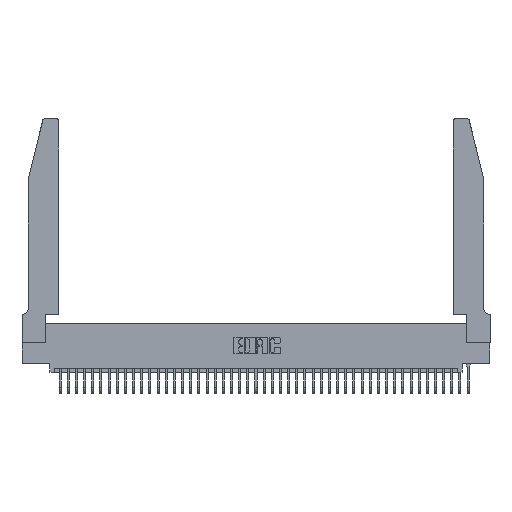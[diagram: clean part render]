
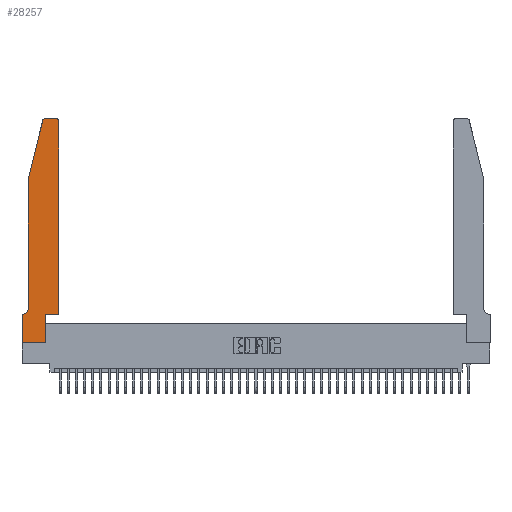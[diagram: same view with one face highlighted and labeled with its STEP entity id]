
A CAD part, top view. The second image highlights one B-rep face of the part: STEP entity #28257.
In plain terms, the highlighted planar face has unit normal (0, 0, 1).
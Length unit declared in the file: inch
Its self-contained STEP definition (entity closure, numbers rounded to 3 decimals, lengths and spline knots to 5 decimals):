
#70 = ORIENTED_EDGE ( 'NONE', *, *, #24352, .T. ) ;
#565 = ORIENTED_EDGE ( 'NONE', *, *, #25854, .T. ) ;
#1243 = VERTEX_POINT ( 'NONE', #2522 ) ;
#1568 = DIRECTION ( 'NONE',  ( 0., 0., 1. ) ) ;
#1955 = CARTESIAN_POINT ( 'NONE',  ( 0., 0., 0.37 ) ) ;
#2493 = VECTOR ( 'NONE', #31071, 39.37008 ) ;
#2522 = CARTESIAN_POINT ( 'NONE',  ( 0.4505, 2.72, 0.37 ) ) ;
#2600 = DIRECTION ( 'NONE',  ( 1., 0., 0. ) ) ;
#3411 = DIRECTION ( 'NONE',  ( 0., 0., -1. ) ) ;
#3461 = CARTESIAN_POINT ( 'NONE',  ( 0.0755, 0.42, 0.37 ) ) ;
#3515 = LINE ( 'NONE', #27961, #2493 ) ;
#3892 = VECTOR ( 'NONE', #11024, 39.37008 ) ;
#4000 = PLANE ( 'NONE',  #39865 ) ;
#5388 = VECTOR ( 'NONE', #6300, 39.37008 ) ;
#5618 = DIRECTION ( 'NONE',  ( 0., -1., 0. ) ) ;
#5879 = EDGE_CURVE ( 'NONE', #16688, #23984, #29863, .T. ) ;
#5885 = VECTOR ( 'NONE', #14058, 39.37008 ) ;
#6300 = DIRECTION ( 'NONE',  ( 1., 0., 0. ) ) ;
#7277 = DIRECTION ( 'NONE',  ( 0., 0., 1. ) ) ;
#7599 = CARTESIAN_POINT ( 'NONE',  ( 0.0755, 0.35, 0.37 ) ) ;
#7938 = EDGE_CURVE ( 'NONE', #16763, #21421, #29204, .T. ) ;
#8326 = ORIENTED_EDGE ( 'NONE', *, *, #30070, .T. ) ;
#8475 = LINE ( 'NONE', #40564, #25289 ) ;
#8668 = DIRECTION ( 'NONE',  ( 0., 1., 0. ) ) ;
#8767 = CARTESIAN_POINT ( 'NONE',  ( 0.0755, 2., 0.37 ) ) ;
#8951 = ORIENTED_EDGE ( 'NONE', *, *, #5879, .T. ) ;
#9298 = ORIENTED_EDGE ( 'NONE', *, *, #7938, .T. ) ;
#9329 = VERTEX_POINT ( 'NONE', #1955 ) ;
#10605 = VECTOR ( 'NONE', #2600, 39.37008 ) ;
#11024 = DIRECTION ( 'NONE',  ( -1., 0., 0. ) ) ;
#12360 = VECTOR ( 'NONE', #36499, 39.37008 ) ;
#12567 = EDGE_CURVE ( 'NONE', #26544, #14189, #13908, .T. ) ;
#13908 = LINE ( 'NONE', #8767, #30537 ) ;
#14058 = DIRECTION ( 'NONE',  ( 0., -1., 0. ) ) ;
#14189 = VERTEX_POINT ( 'NONE', #3461 ) ;
#14202 = VECTOR ( 'NONE', #8668, 39.37008 ) ;
#15134 = DIRECTION ( 'NONE',  ( 0., 0., 1. ) ) ;
#16160 = EDGE_CURVE ( 'NONE', #29964, #26544, #3515, .T. ) ;
#16688 = VERTEX_POINT ( 'NONE', #39646 ) ;
#16763 = VERTEX_POINT ( 'NONE', #27642 ) ;
#16911 = AXIS2_PLACEMENT_3D ( 'NONE', #20706, #1568, #23895 ) ;
#17182 = VERTEX_POINT ( 'NONE', #17239 ) ;
#17239 = CARTESIAN_POINT ( 'NONE',  ( 0.284, 2.75, 0.37 ) ) ;
#17277 = VERTEX_POINT ( 'NONE', #18311 ) ;
#18182 = CARTESIAN_POINT ( 'NONE',  ( 0.25487, 2.72718, 0.37 ) ) ;
#18311 = CARTESIAN_POINT ( 'NONE',  ( 0.4505, 0.35, 0.37 ) ) ;
#18695 = ORIENTED_EDGE ( 'NONE', *, *, #22180, .T. ) ;
#18732 = CARTESIAN_POINT ( 'NONE',  ( 0.4205, 2.75, 0.37 ) ) ;
#18925 = ORIENTED_EDGE ( 'NONE', *, *, #16160, .T. ) ;
#20449 = CARTESIAN_POINT ( 'NONE',  ( 0.0755, 2., 0.37 ) ) ;
#20580 = ORIENTED_EDGE ( 'NONE', *, *, #12567, .T. ) ;
#20706 = CARTESIAN_POINT ( 'NONE',  ( 0.284, 2.72, 0.37 ) ) ;
#20847 = CIRCLE ( 'NONE', #21564, 0.03 ) ;
#21421 = VERTEX_POINT ( 'NONE', #31385 ) ;
#21564 = AXIS2_PLACEMENT_3D ( 'NONE', #33845, #15134, #36988 ) ;
#21856 = DIRECTION ( 'NONE',  ( -1., 0., 0. ) ) ;
#22131 = CARTESIAN_POINT ( 'NONE',  ( 0.4505, 0.35, 0.37 ) ) ;
#22180 = EDGE_CURVE ( 'NONE', #1243, #30088, #20847, .T. ) ;
#22493 = CARTESIAN_POINT ( 'NONE',  ( 0.0055, 0.42, 0.37 ) ) ;
#22948 = CIRCLE ( 'NONE', #35762, 0.07 ) ;
#23326 = LINE ( 'NONE', #22131, #5388 ) ;
#23511 = CARTESIAN_POINT ( 'NONE',  ( 0., 0., 0.37 ) ) ;
#23895 = DIRECTION ( 'NONE',  ( 1., 0., 0. ) ) ;
#23984 = VERTEX_POINT ( 'NONE', #30187 ) ;
#24352 = EDGE_CURVE ( 'NONE', #14189, #16763, #22948, .T. ) ;
#24912 = CARTESIAN_POINT ( 'NONE',  ( 0., 0., 0.37 ) ) ;
#25289 = VECTOR ( 'NONE', #21856, 39.37008 ) ;
#25668 = DIRECTION ( 'NONE',  ( -1., 0., 0. ) ) ;
#25749 = EDGE_CURVE ( 'NONE', #30088, #17182, #8475, .T. ) ;
#25854 = EDGE_CURVE ( 'NONE', #23984, #17277, #23326, .T. ) ;
#25924 = EDGE_LOOP ( 'NONE', ( #37283, #27921, #18925, #20580, #70, #9298, #37052, #8326, #8951, #565, #35861, #18695 ) ) ;
#26044 = EDGE_CURVE ( 'NONE', #21421, #9329, #38443, .T. ) ;
#26286 = CIRCLE ( 'NONE', #16911, 0.03 ) ;
#26544 = VERTEX_POINT ( 'NONE', #20449 ) ;
#27544 = CARTESIAN_POINT ( 'NONE',  ( 0.2865, 0.35, 0.37 ) ) ;
#27642 = CARTESIAN_POINT ( 'NONE',  ( 0.0055, 0.35, 0.37 ) ) ;
#27810 = EDGE_CURVE ( 'NONE', #17277, #1243, #30019, .T. ) ;
#27921 = ORIENTED_EDGE ( 'NONE', *, *, #30973, .T. ) ;
#27961 = CARTESIAN_POINT ( 'NONE',  ( 0.0755, 2., 0.37 ) ) ;
#28257 = ADVANCED_FACE ( 'NONE', ( #36318 ), #4000, .T. ) ;
#28312 = LINE ( 'NONE', #24912, #10605 ) ;
#29204 = LINE ( 'NONE', #7599, #3892 ) ;
#29379 = DIRECTION ( 'NONE',  ( 1., 0., 0. ) ) ;
#29863 = LINE ( 'NONE', #27544, #14202 ) ;
#29964 = VERTEX_POINT ( 'NONE', #18182 ) ;
#30019 = LINE ( 'NONE', #30229, #12360 ) ;
#30070 = EDGE_CURVE ( 'NONE', #9329, #16688, #28312, .T. ) ;
#30088 = VERTEX_POINT ( 'NONE', #18732 ) ;
#30187 = CARTESIAN_POINT ( 'NONE',  ( 0.2865, 0.35, 0.37 ) ) ;
#30229 = CARTESIAN_POINT ( 'NONE',  ( 0.4505, 0.35, 0.37 ) ) ;
#30537 = VECTOR ( 'NONE', #5618, 39.37008 ) ;
#30973 = EDGE_CURVE ( 'NONE', #17182, #29964, #26286, .T. ) ;
#31071 = DIRECTION ( 'NONE',  ( -0.239, -0.971, 0. ) ) ;
#31385 = CARTESIAN_POINT ( 'NONE',  ( 0., 0.35, 0.37 ) ) ;
#33845 = CARTESIAN_POINT ( 'NONE',  ( 0.4205, 2.72, 0.37 ) ) ;
#35762 = AXIS2_PLACEMENT_3D ( 'NONE', #22493, #3411, #25668 ) ;
#35861 = ORIENTED_EDGE ( 'NONE', *, *, #27810, .T. ) ;
#36318 = FACE_OUTER_BOUND ( 'NONE', #25924, .T. ) ;
#36499 = DIRECTION ( 'NONE',  ( 0., 1., 0. ) ) ;
#36988 = DIRECTION ( 'NONE',  ( 1., 0., 0. ) ) ;
#37052 = ORIENTED_EDGE ( 'NONE', *, *, #26044, .T. ) ;
#37283 = ORIENTED_EDGE ( 'NONE', *, *, #25749, .T. ) ;
#38443 = LINE ( 'NONE', #23511, #5885 ) ;
#38671 = CARTESIAN_POINT ( 'NONE',  ( 0., 0.35, 0.37 ) ) ;
#39646 = CARTESIAN_POINT ( 'NONE',  ( 0.2865, 0., 0.37 ) ) ;
#39865 = AXIS2_PLACEMENT_3D ( 'NONE', #38671, #7277, #29379 ) ;
#40564 = CARTESIAN_POINT ( 'NONE',  ( 0.2605, 2.75, 0.37 ) ) ;
